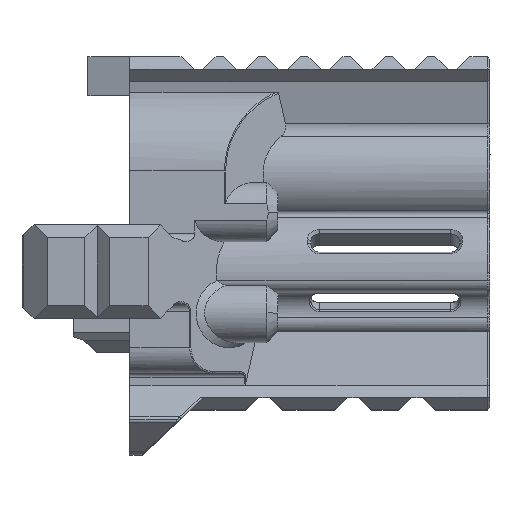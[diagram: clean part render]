
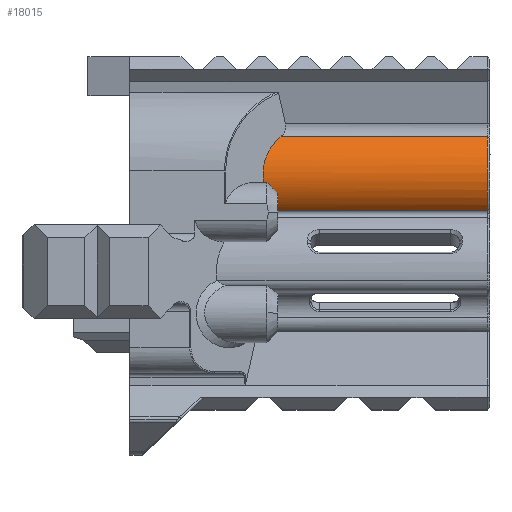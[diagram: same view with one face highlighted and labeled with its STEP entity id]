
A CAD part, top view. The second image highlights one B-rep face of the part: STEP entity #18015.
In plain terms, the highlighted cylindrical face has radius 11.5 mm (diameter 23 mm), a partial arc.
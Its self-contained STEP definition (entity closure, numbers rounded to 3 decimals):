
#71 = CARTESIAN_POINT ( 'NONE',  ( 43.387, 44.223, 11.934 ) ) ;
#458 = CARTESIAN_POINT ( 'NONE',  ( 44.531, 43.706, 11.816 ) ) ;
#676 = CARTESIAN_POINT ( 'NONE',  ( 96.19, 55.535, 7.914 ) ) ;
#922 = AXIS2_PLACEMENT_3D ( 'NONE', #2593, #2291, #17335 ) ;
#1091 = FACE_OUTER_BOUND ( 'NONE', #19030, .T. ) ;
#1101 = CARTESIAN_POINT ( 'NONE',  ( 47.407, 55.535, 7.914 ) ) ;
#1416 = CARTESIAN_POINT ( 'NONE',  ( 43.958, 52.745, 11.363 ) ) ;
#1464 = VERTEX_POINT ( 'NONE', #10131 ) ;
#1698 = ORIENTED_EDGE ( 'NONE', *, *, #12540, .T. ) ;
#1764 = CARTESIAN_POINT ( 'NONE',  ( 46.265, 40.354, 10.346 ) ) ;
#2047 = CARTESIAN_POINT ( 'NONE',  ( 45.519, 42.371, 11.381 ) ) ;
#2291 = DIRECTION ( 'NONE',  ( -1., 0., 0. ) ) ;
#2593 = CARTESIAN_POINT ( 'NONE',  ( 45.79, 46.595, 0.681 ) ) ;
#2810 = ORIENTED_EDGE ( 'NONE', *, *, #18342, .F. ) ;
#3341 = CARTESIAN_POINT ( 'NONE',  ( 44.092, 44.223, 11.934 ) ) ;
#3848 = DIRECTION ( 'NONE',  ( 1., 0., 0. ) ) ;
#4115 = CIRCLE ( 'NONE', #10108, 11.5 ) ;
#4643 = CARTESIAN_POINT ( 'NONE',  ( 45.23, 38.178, 8.523 ) ) ;
#4934 = CARTESIAN_POINT ( 'NONE',  ( 44.949, 43.18, 11.666 ) ) ;
#5224 = VECTOR ( 'NONE', #8420, 1000. ) ;
#5538 = ORIENTED_EDGE ( 'NONE', *, *, #13297, .F. ) ;
#5567 = CARTESIAN_POINT ( 'NONE',  ( 96.19, 46.595, 0.681 ) ) ;
#5783 = VERTEX_POINT ( 'NONE', #1101 ) ;
#5829 = CARTESIAN_POINT ( 'NONE',  ( 46.196, 39.795, 9.957 ) ) ;
#6175 = ORIENTED_EDGE ( 'NONE', *, *, #12090, .T. ) ;
#6218 = EDGE_CURVE ( 'NONE', #12482, #5783, #16228, .T. ) ;
#6612 = CARTESIAN_POINT ( 'NONE',  ( 46.223, 39.932, 10.056 ) ) ;
#6952 = CYLINDRICAL_SURFACE ( 'NONE', #922, 11.5 ) ;
#7350 = DIRECTION ( 'NONE',  ( 1., 0., 0. ) ) ;
#7471 = CARTESIAN_POINT ( 'NONE',  ( 42.472, 48.564, 12.849 ) ) ;
#7515 = CARTESIAN_POINT ( 'NONE',  ( 45.749, 38.798, 9.14 ) ) ;
#7564 = ORIENTED_EDGE ( 'NONE', *, *, #18882, .F. ) ;
#8323 = CARTESIAN_POINT ( 'NONE',  ( 36.678, 44.223, 11.934 ) ) ;
#8420 = DIRECTION ( 'NONE',  ( -1., 0., 0. ) ) ;
#8931 = CARTESIAN_POINT ( 'NONE',  ( 47.407, 55.535, 7.914 ) ) ;
#8977 = CARTESIAN_POINT ( 'NONE',  ( 45.032, 37.993, 8.314 ) ) ;
#9429 = B_SPLINE_CURVE_WITH_KNOTS ( 'NONE', 3,
 ( #8977, #4643, #13338, #7515, #19380, #13538, #18196, #5829, #6612, #1764, #12531, #10757, #9655, #16805, #2047, #14015, #4934, #458, #10947, #3341 ),
 .UNSPECIFIED., .F., .F.,
 ( 4, 2, 2, 2, 2, 2, 2, 2, 2, 4 ),
 ( 0., 0.001, 0.002, 0.003, 0.003, 0.004, 0.005, 0.006, 0.007, 0.008 ),
 .UNSPECIFIED. ) ;
#9655 = CARTESIAN_POINT ( 'NONE',  ( 45.977, 41.529, 11.01 ) ) ;
#9722 = VERTEX_POINT ( 'NONE', #9794 ) ;
#9794 = CARTESIAN_POINT ( 'NONE',  ( 96.19, 37.993, 8.314 ) ) ;
#10108 = AXIS2_PLACEMENT_3D ( 'NONE', #5567, #7350, #11589 ) ;
#10131 = CARTESIAN_POINT ( 'NONE',  ( 45.032, 37.993, 8.314 ) ) ;
#10583 = VECTOR ( 'NONE', #3848, 1000. ) ;
#10757 = CARTESIAN_POINT ( 'NONE',  ( 46.096, 41.236, 10.862 ) ) ;
#10901 = VECTOR ( 'NONE', #12857, 1000. ) ;
#10947 = CARTESIAN_POINT ( 'NONE',  ( 44.314, 43.966, 11.88 ) ) ;
#11170 =( BOUNDED_CURVE ( )  B_SPLINE_CURVE ( 3, ( #8931, #1416, #7471, #13292 ),
 .UNSPECIFIED., .F., .T. ) 
 B_SPLINE_CURVE_WITH_KNOTS ( ( 4, 4 ),
 ( 5.393, 6.491 ),
 .UNSPECIFIED. ) 
 CURVE ( )  GEOMETRIC_REPRESENTATION_ITEM ( )  RATIONAL_B_SPLINE_CURVE ( ( 1., 0.902, 0.902, 1. ) ) 
 REPRESENTATION_ITEM ( '' )  );
#11356 = LINE ( 'NONE', #17404, #10583 ) ;
#11574 = CARTESIAN_POINT ( 'NONE',  ( 45.79, 55.535, 7.914 ) ) ;
#11589 = DIRECTION ( 'NONE',  ( 0., 0., 1. ) ) ;
#12090 = EDGE_CURVE ( 'NONE', #5783, #15750, #11170, .T. ) ;
#12482 = VERTEX_POINT ( 'NONE', #676 ) ;
#12531 = CARTESIAN_POINT ( 'NONE',  ( 46.24, 40.652, 10.532 ) ) ;
#12540 = EDGE_CURVE ( 'NONE', #1464, #9722, #11356, .T. ) ;
#12857 = DIRECTION ( 'NONE',  ( -1., 0., 0. ) ) ;
#13292 = CARTESIAN_POINT ( 'NONE',  ( 43.387, 44.223, 11.934 ) ) ;
#13297 = EDGE_CURVE ( 'NONE', #15941, #15750, #18627, .T. ) ;
#13338 = CARTESIAN_POINT ( 'NONE',  ( 45.416, 38.375, 8.729 ) ) ;
#13538 = CARTESIAN_POINT ( 'NONE',  ( 46.07, 39.396, 9.651 ) ) ;
#14015 = CARTESIAN_POINT ( 'NONE',  ( 45.149, 42.913, 11.58 ) ) ;
#15368 = ORIENTED_EDGE ( 'NONE', *, *, #6218, .T. ) ;
#15750 = VERTEX_POINT ( 'NONE', #71 ) ;
#15941 = VERTEX_POINT ( 'NONE', #16391 ) ;
#16228 = LINE ( 'NONE', #11574, #5224 ) ;
#16391 = CARTESIAN_POINT ( 'NONE',  ( 44.092, 44.223, 11.934 ) ) ;
#16805 = CARTESIAN_POINT ( 'NONE',  ( 45.689, 42.096, 11.269 ) ) ;
#17335 = DIRECTION ( 'NONE',  ( 0., -1., 0. ) ) ;
#17404 = CARTESIAN_POINT ( 'NONE',  ( 45.79, 37.993, 8.314 ) ) ;
#18015 = ADVANCED_FACE ( 'NONE', ( #1091 ), #6952, .T. ) ;
#18196 = CARTESIAN_POINT ( 'NONE',  ( 46.12, 39.527, 9.754 ) ) ;
#18342 = EDGE_CURVE ( 'NONE', #1464, #15941, #9429, .T. ) ;
#18627 = LINE ( 'NONE', #8323, #10901 ) ;
#18882 = EDGE_CURVE ( 'NONE', #12482, #9722, #4115, .T. ) ;
#19030 = EDGE_LOOP ( 'NONE', ( #2810, #1698, #7564, #15368, #6175, #5538 ) ) ;
#19380 = CARTESIAN_POINT ( 'NONE',  ( 45.897, 39.024, 9.344 ) ) ;
